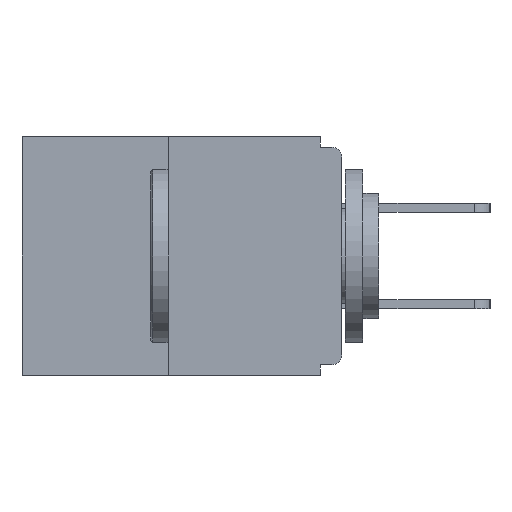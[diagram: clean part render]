
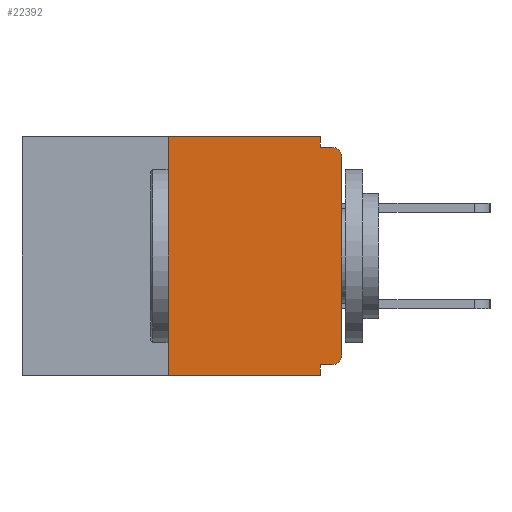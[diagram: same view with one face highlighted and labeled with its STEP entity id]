
A CAD part, left-side view. The second image highlights one B-rep face of the part: STEP entity #22392.
In plain terms, the highlighted planar face has unit normal (-1, 0, 0).
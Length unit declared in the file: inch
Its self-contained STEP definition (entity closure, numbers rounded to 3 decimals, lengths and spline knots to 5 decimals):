
#777 = EDGE_LOOP ( 'NONE', ( #11764, #1630, #16661, #2274, #15512, #23518, #11257, #13390, #23350, #21618 ) ) ;
#1630 = ORIENTED_EDGE ( 'NONE', *, *, #19252, .F. ) ;
#1855 = VECTOR ( 'NONE', #6940, 39.37008 ) ;
#1924 = CARTESIAN_POINT ( 'NONE',  ( 0., 0.46, -0.343 ) ) ;
#1965 = LINE ( 'NONE', #17841, #18395 ) ;
#2274 = ORIENTED_EDGE ( 'NONE', *, *, #21240, .F. ) ;
#2342 = EDGE_CURVE ( 'NONE', #21530, #13548, #1965, .T. ) ;
#2365 = CARTESIAN_POINT ( 'NONE',  ( 0., 0.46, 0. ) ) ;
#2848 = VECTOR ( 'NONE', #15031, 39.37008 ) ;
#2923 = CARTESIAN_POINT ( 'NONE',  ( 0., 0.031, 0. ) ) ;
#3089 = DIRECTION ( 'NONE',  ( 0., 1., 0. ) ) ;
#3144 = VERTEX_POINT ( 'NONE', #13781 ) ;
#3255 = CARTESIAN_POINT ( 'NONE',  ( 0., 0., -0.328 ) ) ;
#3282 = AXIS2_PLACEMENT_3D ( 'NONE', #4693, #12408, #8718 ) ;
#3788 = CARTESIAN_POINT ( 'NONE',  ( 0., 0.25, 0. ) ) ;
#3838 = CARTESIAN_POINT ( 'NONE',  ( 0., 0.25, -0.343 ) ) ;
#4347 = EDGE_CURVE ( 'NONE', #17490, #21530, #16236, .T. ) ;
#4588 = CIRCLE ( 'NONE', #13907, 0.015 ) ;
#4693 = CARTESIAN_POINT ( 'NONE',  ( 0., 0.46, 0. ) ) ;
#5094 = DIRECTION ( 'NONE',  ( 0., 0., -1. ) ) ;
#5151 = CARTESIAN_POINT ( 'NONE',  ( 0., 0.015, -0.328 ) ) ;
#5835 = EDGE_CURVE ( 'NONE', #21192, #13548, #4588, .T. ) ;
#6224 = EDGE_CURVE ( 'NONE', #20895, #17490, #8693, .T. ) ;
#6791 = VECTOR ( 'NONE', #3089, 39.37008 ) ;
#6940 = DIRECTION ( 'NONE',  ( 0., 0., -1. ) ) ;
#7136 = DIRECTION ( 'NONE',  ( 0., 0., -1. ) ) ;
#8025 = DIRECTION ( 'NONE',  ( 0., -1., 0. ) ) ;
#8427 = LINE ( 'NONE', #1924, #2848 ) ;
#8529 = EDGE_CURVE ( 'NONE', #9948, #14213, #13553, .T. ) ;
#8693 = LINE ( 'NONE', #2365, #11042 ) ;
#8718 = DIRECTION ( 'NONE',  ( 0., 0., -1. ) ) ;
#9151 = LINE ( 'NONE', #3255, #6791 ) ;
#9948 = VERTEX_POINT ( 'NONE', #5151 ) ;
#10206 = CARTESIAN_POINT ( 'NONE',  ( 0., 0., -0.313 ) ) ;
#10340 = CARTESIAN_POINT ( 'NONE',  ( 0., 0.031, 0. ) ) ;
#10419 = CARTESIAN_POINT ( 'NONE',  ( 0., 0.015, -0.03 ) ) ;
#11042 = VECTOR ( 'NONE', #8025, 39.37008 ) ;
#11257 = ORIENTED_EDGE ( 'NONE', *, *, #13780, .T. ) ;
#11323 = VECTOR ( 'NONE', #11892, 39.37008 ) ;
#11633 = CARTESIAN_POINT ( 'NONE',  ( 0., 0.031, -0.015 ) ) ;
#11736 = CARTESIAN_POINT ( 'NONE',  ( 0., 0.25, 0. ) ) ;
#11764 = ORIENTED_EDGE ( 'NONE', *, *, #6224, .F. ) ;
#11892 = DIRECTION ( 'NONE',  ( 0., 0., 1. ) ) ;
#12408 = DIRECTION ( 'NONE',  ( 1., 0., 0. ) ) ;
#12909 = FACE_OUTER_BOUND ( 'NONE', #777, .T. ) ;
#12955 = CARTESIAN_POINT ( 'NONE',  ( 0., 0., -0.03 ) ) ;
#13390 = ORIENTED_EDGE ( 'NONE', *, *, #5835, .T. ) ;
#13548 = VERTEX_POINT ( 'NONE', #19136 ) ;
#13553 = CIRCLE ( 'NONE', #17151, 0.015 ) ;
#13780 = EDGE_CURVE ( 'NONE', #14213, #21192, #18282, .T. ) ;
#13781 = CARTESIAN_POINT ( 'NONE',  ( 0., 0.031, -0.328 ) ) ;
#13907 = AXIS2_PLACEMENT_3D ( 'NONE', #10419, #17910, #5094 ) ;
#14213 = VERTEX_POINT ( 'NONE', #10206 ) ;
#15031 = DIRECTION ( 'NONE',  ( 0., -1., 0. ) ) ;
#15512 = ORIENTED_EDGE ( 'NONE', *, *, #21816, .F. ) ;
#16236 = LINE ( 'NONE', #2923, #1855 ) ;
#16322 = LINE ( 'NONE', #11736, #11323 ) ;
#16562 = VERTEX_POINT ( 'NONE', #3838 ) ;
#16661 = ORIENTED_EDGE ( 'NONE', *, *, #17246, .T. ) ;
#17151 = AXIS2_PLACEMENT_3D ( 'NONE', #22860, #21136, #17370 ) ;
#17246 = EDGE_CURVE ( 'NONE', #16562, #17919, #8427, .T. ) ;
#17370 = DIRECTION ( 'NONE',  ( 0., 0., -1. ) ) ;
#17490 = VERTEX_POINT ( 'NONE', #10340 ) ;
#17763 = DIRECTION ( 'NONE',  ( 0., -1., 0. ) ) ;
#17841 = CARTESIAN_POINT ( 'NONE',  ( 0., 0., -0.015 ) ) ;
#17910 = DIRECTION ( 'NONE',  ( -1., 0., 0. ) ) ;
#17919 = VERTEX_POINT ( 'NONE', #22817 ) ;
#18002 = PLANE ( 'NONE',  #3282 ) ;
#18263 = VECTOR ( 'NONE', #7136, 39.37008 ) ;
#18282 = LINE ( 'NONE', #20545, #20667 ) ;
#18395 = VECTOR ( 'NONE', #17763, 39.37008 ) ;
#19136 = CARTESIAN_POINT ( 'NONE',  ( 0., 0.015, -0.015 ) ) ;
#19252 = EDGE_CURVE ( 'NONE', #16562, #20895, #16322, .T. ) ;
#20376 = DIRECTION ( 'NONE',  ( 0., 0., 1. ) ) ;
#20545 = CARTESIAN_POINT ( 'NONE',  ( 0., 0., 0. ) ) ;
#20667 = VECTOR ( 'NONE', #20376, 39.37008 ) ;
#20895 = VERTEX_POINT ( 'NONE', #3788 ) ;
#21136 = DIRECTION ( 'NONE',  ( -1., 0., 0. ) ) ;
#21192 = VERTEX_POINT ( 'NONE', #12955 ) ;
#21240 = EDGE_CURVE ( 'NONE', #3144, #17919, #21489, .T. ) ;
#21489 = LINE ( 'NONE', #24229, #18263 ) ;
#21530 = VERTEX_POINT ( 'NONE', #11633 ) ;
#21618 = ORIENTED_EDGE ( 'NONE', *, *, #4347, .F. ) ;
#21816 = EDGE_CURVE ( 'NONE', #9948, #3144, #9151, .T. ) ;
#22392 = ADVANCED_FACE ( 'NONE', ( #12909 ), #18002, .F. ) ;
#22817 = CARTESIAN_POINT ( 'NONE',  ( 0., 0.031, -0.343 ) ) ;
#22860 = CARTESIAN_POINT ( 'NONE',  ( 0., 0.015, -0.313 ) ) ;
#23350 = ORIENTED_EDGE ( 'NONE', *, *, #2342, .F. ) ;
#23518 = ORIENTED_EDGE ( 'NONE', *, *, #8529, .T. ) ;
#24229 = CARTESIAN_POINT ( 'NONE',  ( 0., 0.031, -0.343 ) ) ;
